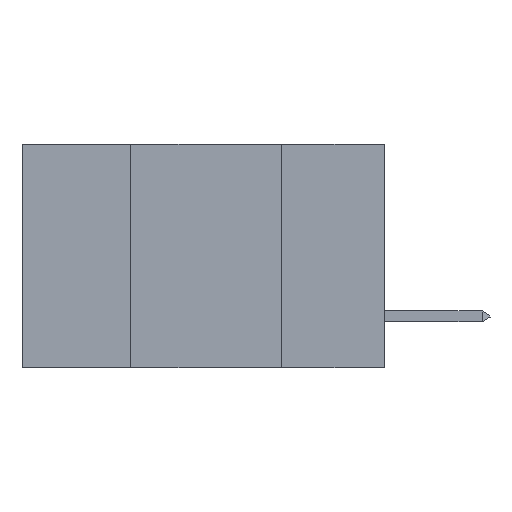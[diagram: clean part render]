
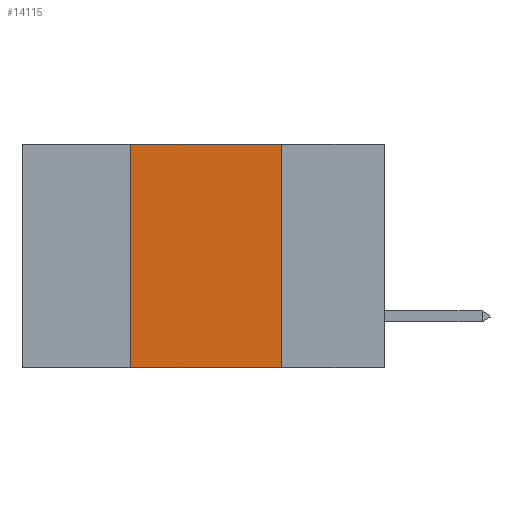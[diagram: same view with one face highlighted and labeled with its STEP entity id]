
A CAD part, left-side view. The second image highlights one B-rep face of the part: STEP entity #14115.
In plain terms, the highlighted planar face has unit normal (-1, 0, 0).
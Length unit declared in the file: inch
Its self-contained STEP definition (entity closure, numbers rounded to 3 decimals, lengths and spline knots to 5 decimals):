
#217 = AXIS2_PLACEMENT_3D ( 'NONE', #16605, #31765, #11861 ) ;
#594 = LINE ( 'NONE', #12944, #12691 ) ;
#1944 = DIRECTION ( 'NONE',  ( 0., -1., 0. ) ) ;
#1955 = VERTEX_POINT ( 'NONE', #10684 ) ;
#4044 = VERTEX_POINT ( 'NONE', #18119 ) ;
#4767 = EDGE_CURVE ( 'NONE', #41416, #4044, #45265, .T. ) ;
#5581 = VERTEX_POINT ( 'NONE', #35159 ) ;
#10640 = VECTOR ( 'NONE', #1944, 39.37008 ) ;
#10684 = CARTESIAN_POINT ( 'NONE',  ( 0., 0.17, 0. ) ) ;
#11861 = DIRECTION ( 'NONE',  ( 0., 0., -1. ) ) ;
#12691 = VECTOR ( 'NONE', #30414, 39.37008 ) ;
#12944 = CARTESIAN_POINT ( 'NONE',  ( 0., 0.17, 0. ) ) ;
#13078 = PLANE ( 'NONE',  #217 ) ;
#13740 = DIRECTION ( 'NONE',  ( 0., -1., 0. ) ) ;
#14115 = ADVANCED_FACE ( 'NONE', ( #16038 ), #13078, .F. ) ;
#15118 = ORIENTED_EDGE ( 'NONE', *, *, #4767, .T. ) ;
#16038 = FACE_OUTER_BOUND ( 'NONE', #29490, .T. ) ;
#16605 = CARTESIAN_POINT ( 'NONE',  ( 0., 0.6, 0. ) ) ;
#18119 = CARTESIAN_POINT ( 'NONE',  ( 0., 0.17, -0.37 ) ) ;
#20478 = ORIENTED_EDGE ( 'NONE', *, *, #37881, .F. ) ;
#20739 = CARTESIAN_POINT ( 'NONE',  ( 0., 0.6, -0.37 ) ) ;
#20918 = DIRECTION ( 'NONE',  ( 0., 0., 1. ) ) ;
#21144 = VECTOR ( 'NONE', #20918, 39.37008 ) ;
#23706 = CARTESIAN_POINT ( 'NONE',  ( 0., 0.42, 0. ) ) ;
#25128 = EDGE_CURVE ( 'NONE', #41416, #5581, #27198, .T. ) ;
#26189 = CARTESIAN_POINT ( 'NONE',  ( 0., 0.42, -0.37 ) ) ;
#27086 = LINE ( 'NONE', #32788, #10640 ) ;
#27198 = LINE ( 'NONE', #23706, #21144 ) ;
#29172 = EDGE_CURVE ( 'NONE', #5581, #1955, #27086, .T. ) ;
#29490 = EDGE_LOOP ( 'NONE', ( #20478, #35188, #42442, #15118 ) ) ;
#30414 = DIRECTION ( 'NONE',  ( 0., 0., -1. ) ) ;
#31765 = DIRECTION ( 'NONE',  ( 1., 0., 0. ) ) ;
#32788 = CARTESIAN_POINT ( 'NONE',  ( 0., 0.6, 0. ) ) ;
#35159 = CARTESIAN_POINT ( 'NONE',  ( 0., 0.42, 0. ) ) ;
#35188 = ORIENTED_EDGE ( 'NONE', *, *, #29172, .F. ) ;
#35914 = VECTOR ( 'NONE', #13740, 39.37008 ) ;
#37881 = EDGE_CURVE ( 'NONE', #1955, #4044, #594, .T. ) ;
#41416 = VERTEX_POINT ( 'NONE', #26189 ) ;
#42442 = ORIENTED_EDGE ( 'NONE', *, *, #25128, .F. ) ;
#45265 = LINE ( 'NONE', #20739, #35914 ) ;
